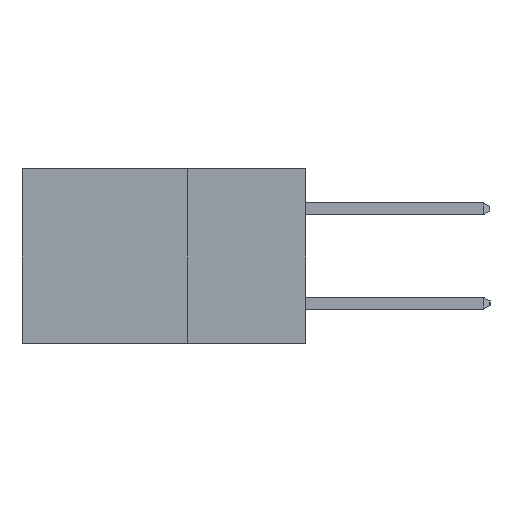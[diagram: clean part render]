
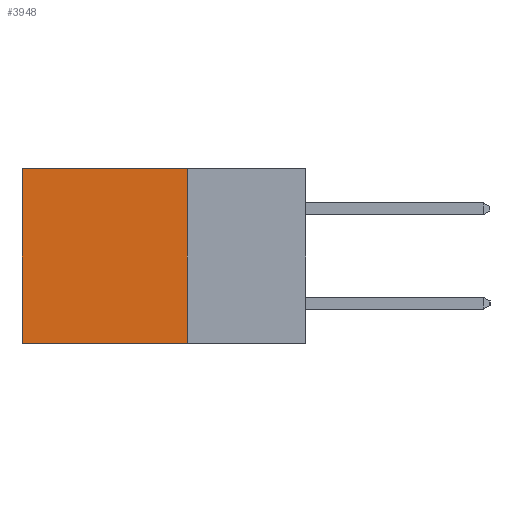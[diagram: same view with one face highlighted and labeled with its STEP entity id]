
A CAD part, left-side view. The second image highlights one B-rep face of the part: STEP entity #3948.
In plain terms, the highlighted planar face has unit normal (-1, 0, 0).
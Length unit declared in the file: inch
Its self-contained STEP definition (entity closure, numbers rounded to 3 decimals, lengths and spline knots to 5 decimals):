
#45 = DIRECTION ( 'NONE',  ( 0., 0., -1. ) ) ;
#717 = CARTESIAN_POINT ( 'NONE',  ( 0.2615, 0.25, -0.37 ) ) ;
#2226 = AXIS2_PLACEMENT_3D ( 'NONE', #12018, #6363, #45 ) ;
#2318 = CARTESIAN_POINT ( 'NONE',  ( 0.2615, 0.6, 0. ) ) ;
#2358 = CARTESIAN_POINT ( 'NONE',  ( 0.2615, 0.6, -0.37 ) ) ;
#2442 = VERTEX_POINT ( 'NONE', #10048 ) ;
#2800 = EDGE_CURVE ( 'NONE', #9281, #10180, #6952, .T. ) ;
#3522 = CARTESIAN_POINT ( 'NONE',  ( 0.2615, 0.25, -0.37 ) ) ;
#3926 = DIRECTION ( 'NONE',  ( 0., 0., -1. ) ) ;
#3940 = CARTESIAN_POINT ( 'NONE',  ( 0.2615, 0.25, 0. ) ) ;
#3948 = ADVANCED_FACE ( 'NONE', ( #12736 ), #6313, .F. ) ;
#4050 = ORIENTED_EDGE ( 'NONE', *, *, #2800, .T. ) ;
#4062 = CARTESIAN_POINT ( 'NONE',  ( 0.2615, 0.25, -0.37 ) ) ;
#4086 = LINE ( 'NONE', #2358, #6478 ) ;
#4341 = CARTESIAN_POINT ( 'NONE',  ( 0.2615, 0.25, 0. ) ) ;
#4420 = LINE ( 'NONE', #3522, #9328 ) ;
#4553 = DIRECTION ( 'NONE',  ( 0., 1., 0. ) ) ;
#5312 = VERTEX_POINT ( 'NONE', #4062 ) ;
#5485 = ORIENTED_EDGE ( 'NONE', *, *, #8564, .F. ) ;
#5811 = ORIENTED_EDGE ( 'NONE', *, *, #6970, .F. ) ;
#6313 = PLANE ( 'NONE',  #2226 ) ;
#6363 = DIRECTION ( 'NONE',  ( 1., 0., 0. ) ) ;
#6478 = VECTOR ( 'NONE', #10333, 39.37008 ) ;
#6504 = EDGE_LOOP ( 'NONE', ( #7507, #5485, #5811, #4050 ) ) ;
#6952 = LINE ( 'NONE', #3940, #9193 ) ;
#6970 = EDGE_CURVE ( 'NONE', #9281, #5312, #11094, .T. ) ;
#7507 = ORIENTED_EDGE ( 'NONE', *, *, #7667, .T. ) ;
#7667 = EDGE_CURVE ( 'NONE', #10180, #2442, #4086, .T. ) ;
#8564 = EDGE_CURVE ( 'NONE', #5312, #2442, #4420, .T. ) ;
#8599 = VECTOR ( 'NONE', #3926, 39.37008 ) ;
#9193 = VECTOR ( 'NONE', #9779, 39.37008 ) ;
#9281 = VERTEX_POINT ( 'NONE', #4341 ) ;
#9328 = VECTOR ( 'NONE', #4553, 39.37008 ) ;
#9779 = DIRECTION ( 'NONE',  ( 0., 1., 0. ) ) ;
#10048 = CARTESIAN_POINT ( 'NONE',  ( 0.2615, 0.6, -0.37 ) ) ;
#10180 = VERTEX_POINT ( 'NONE', #2318 ) ;
#10333 = DIRECTION ( 'NONE',  ( 0., 0., -1. ) ) ;
#11094 = LINE ( 'NONE', #717, #8599 ) ;
#12018 = CARTESIAN_POINT ( 'NONE',  ( 0.2615, 0.25, -0.37 ) ) ;
#12736 = FACE_OUTER_BOUND ( 'NONE', #6504, .T. ) ;
